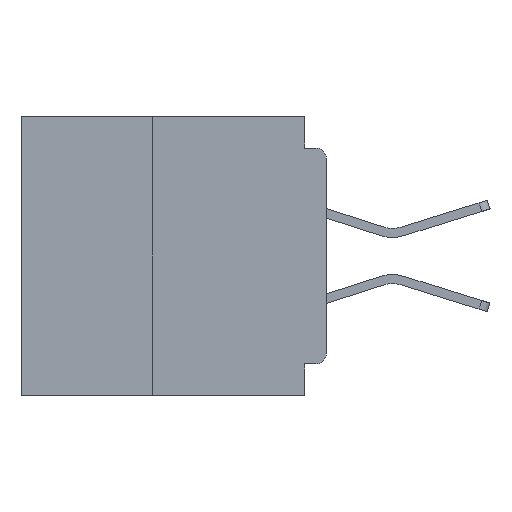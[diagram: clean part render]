
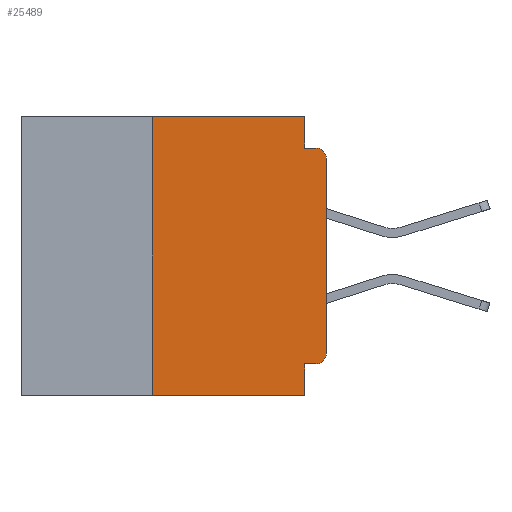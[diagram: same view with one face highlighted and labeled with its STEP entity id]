
A CAD part, left-side view. The second image highlights one B-rep face of the part: STEP entity #25489.
In plain terms, the highlighted planar face has unit normal (-1, 0, 0).
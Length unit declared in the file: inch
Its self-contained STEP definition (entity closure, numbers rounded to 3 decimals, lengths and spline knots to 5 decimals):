
#213 = CARTESIAN_POINT ( 'NONE',  ( 0., 0., 0. ) ) ;
#645 = DIRECTION ( 'NONE',  ( 0., -1., 0. ) ) ;
#1510 = VECTOR ( 'NONE', #11663, 39.37008 ) ;
#2264 = LINE ( 'NONE', #62536, #29198 ) ;
#2270 = DIRECTION ( 'NONE',  ( 0., 0., 1. ) ) ;
#3946 = ORIENTED_EDGE ( 'NONE', *, *, #38854, .F. ) ;
#4465 = LINE ( 'NONE', #52560, #57837 ) ;
#4497 = CARTESIAN_POINT ( 'NONE',  ( 0., 0.437, 0. ) ) ;
#5372 = LINE ( 'NONE', #213, #30723 ) ;
#5453 = LINE ( 'NONE', #36045, #42560 ) ;
#5520 = DIRECTION ( 'NONE',  ( 0., 0., 1. ) ) ;
#6665 = DIRECTION ( 'NONE',  ( 0., -1., 0. ) ) ;
#7525 = EDGE_CURVE ( 'NONE', #46147, #50936, #2264, .T. ) ;
#7867 = FACE_OUTER_BOUND ( 'NONE', #21972, .T. ) ;
#7905 = EDGE_CURVE ( 'NONE', #62162, #35605, #5372, .T. ) ;
#8663 = CARTESIAN_POINT ( 'NONE',  ( 0., 0.015, -0.355 ) ) ;
#9620 = PLANE ( 'NONE',  #54776 ) ;
#9899 = LINE ( 'NONE', #36950, #48418 ) ;
#10013 = EDGE_CURVE ( 'NONE', #64572, #46147, #25686, .T. ) ;
#11040 = ORIENTED_EDGE ( 'NONE', *, *, #27993, .F. ) ;
#11663 = DIRECTION ( 'NONE',  ( 0., 0., -1. ) ) ;
#12031 = CARTESIAN_POINT ( 'NONE',  ( 0., 0.25, 0. ) ) ;
#12203 = CARTESIAN_POINT ( 'NONE',  ( 0., 0., -0.34 ) ) ;
#12264 = VECTOR ( 'NONE', #20190, 39.37008 ) ;
#13597 = EDGE_CURVE ( 'NONE', #22623, #23956, #44892, .T. ) ;
#13922 = VERTEX_POINT ( 'NONE', #60150 ) ;
#14695 = DIRECTION ( 'NONE',  ( 0., 0., -1. ) ) ;
#15246 = CIRCLE ( 'NONE', #57712, 0.015 ) ;
#15384 = CARTESIAN_POINT ( 'NONE',  ( 0., 0.015, -0.34 ) ) ;
#16703 = CARTESIAN_POINT ( 'NONE',  ( 0., 0.031, -0.4 ) ) ;
#16795 = VERTEX_POINT ( 'NONE', #8663 ) ;
#20190 = DIRECTION ( 'NONE',  ( 0., 0., -1. ) ) ;
#20462 = DIRECTION ( 'NONE',  ( 0., 0., -1. ) ) ;
#21972 = EDGE_LOOP ( 'NONE', ( #50018, #36908, #22794, #48707, #11040, #53387, #62722, #29278, #3946, #35606 ) ) ;
#22623 = VERTEX_POINT ( 'NONE', #32677 ) ;
#22794 = ORIENTED_EDGE ( 'NONE', *, *, #7525, .F. ) ;
#23956 = VERTEX_POINT ( 'NONE', #12031 ) ;
#25489 = ADVANCED_FACE ( 'NONE', ( #7867 ), #9620, .F. ) ;
#25686 = LINE ( 'NONE', #35231, #12264 ) ;
#27993 = EDGE_CURVE ( 'NONE', #23956, #64572, #5453, .T. ) ;
#29198 = VECTOR ( 'NONE', #37852, 39.37008 ) ;
#29278 = ORIENTED_EDGE ( 'NONE', *, *, #47475, .F. ) ;
#29450 = CARTESIAN_POINT ( 'NONE',  ( 0., 0.015, -0.06 ) ) ;
#29933 = CARTESIAN_POINT ( 'NONE',  ( 0., 0.031, 0. ) ) ;
#30468 = AXIS2_PLACEMENT_3D ( 'NONE', #29450, #64224, #34528 ) ;
#30504 = EDGE_CURVE ( 'NONE', #22623, #13922, #9899, .T. ) ;
#30723 = VECTOR ( 'NONE', #5520, 39.37008 ) ;
#31597 = VECTOR ( 'NONE', #2270, 39.37008 ) ;
#32677 = CARTESIAN_POINT ( 'NONE',  ( 0., 0.25, -0.4 ) ) ;
#34528 = DIRECTION ( 'NONE',  ( 0., 0., -1. ) ) ;
#35231 = CARTESIAN_POINT ( 'NONE',  ( 0., 0.031, 0. ) ) ;
#35564 = EDGE_CURVE ( 'NONE', #16795, #62162, #15246, .T. ) ;
#35606 = ORIENTED_EDGE ( 'NONE', *, *, #35564, .T. ) ;
#35605 = VERTEX_POINT ( 'NONE', #55435 ) ;
#36045 = CARTESIAN_POINT ( 'NONE',  ( 0., 0.437, 0. ) ) ;
#36403 = CARTESIAN_POINT ( 'NONE',  ( 0., 0.031, -0.045 ) ) ;
#36908 = ORIENTED_EDGE ( 'NONE', *, *, #52649, .T. ) ;
#36950 = CARTESIAN_POINT ( 'NONE',  ( 0., 0.437, -0.4 ) ) ;
#37480 = CARTESIAN_POINT ( 'NONE',  ( 0., 0.031, -0.355 ) ) ;
#37640 = DIRECTION ( 'NONE',  ( 0., 1., 0. ) ) ;
#37852 = DIRECTION ( 'NONE',  ( 0., -1., 0. ) ) ;
#38854 = EDGE_CURVE ( 'NONE', #16795, #53642, #4465, .T. ) ;
#42560 = VECTOR ( 'NONE', #645, 39.37008 ) ;
#42651 = CARTESIAN_POINT ( 'NONE',  ( 0., 0.25, -0.4 ) ) ;
#43749 = CIRCLE ( 'NONE', #30468, 0.015 ) ;
#44892 = LINE ( 'NONE', #42651, #31597 ) ;
#46147 = VERTEX_POINT ( 'NONE', #36403 ) ;
#47475 = EDGE_CURVE ( 'NONE', #53642, #13922, #54921, .T. ) ;
#48418 = VECTOR ( 'NONE', #6665, 39.37008 ) ;
#48707 = ORIENTED_EDGE ( 'NONE', *, *, #10013, .F. ) ;
#49553 = DIRECTION ( 'NONE',  ( 1., 0., 0. ) ) ;
#50018 = ORIENTED_EDGE ( 'NONE', *, *, #7905, .T. ) ;
#50472 = DIRECTION ( 'NONE',  ( -1., 0., 0. ) ) ;
#50936 = VERTEX_POINT ( 'NONE', #53270 ) ;
#52560 = CARTESIAN_POINT ( 'NONE',  ( 0., 0., -0.355 ) ) ;
#52649 = EDGE_CURVE ( 'NONE', #35605, #50936, #43749, .T. ) ;
#53270 = CARTESIAN_POINT ( 'NONE',  ( 0., 0.015, -0.045 ) ) ;
#53387 = ORIENTED_EDGE ( 'NONE', *, *, #13597, .F. ) ;
#53642 = VERTEX_POINT ( 'NONE', #37480 ) ;
#54776 = AXIS2_PLACEMENT_3D ( 'NONE', #4497, #49553, #14695 ) ;
#54921 = LINE ( 'NONE', #16703, #1510 ) ;
#55435 = CARTESIAN_POINT ( 'NONE',  ( 0., 0., -0.06 ) ) ;
#57712 = AXIS2_PLACEMENT_3D ( 'NONE', #15384, #50472, #20462 ) ;
#57837 = VECTOR ( 'NONE', #37640, 39.37008 ) ;
#60150 = CARTESIAN_POINT ( 'NONE',  ( 0., 0.031, -0.4 ) ) ;
#62162 = VERTEX_POINT ( 'NONE', #12203 ) ;
#62536 = CARTESIAN_POINT ( 'NONE',  ( 0., 0., -0.045 ) ) ;
#62722 = ORIENTED_EDGE ( 'NONE', *, *, #30504, .T. ) ;
#64224 = DIRECTION ( 'NONE',  ( -1., 0., 0. ) ) ;
#64572 = VERTEX_POINT ( 'NONE', #29933 ) ;
